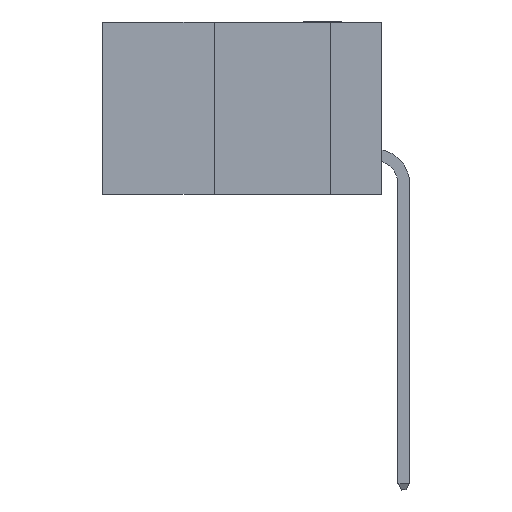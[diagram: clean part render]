
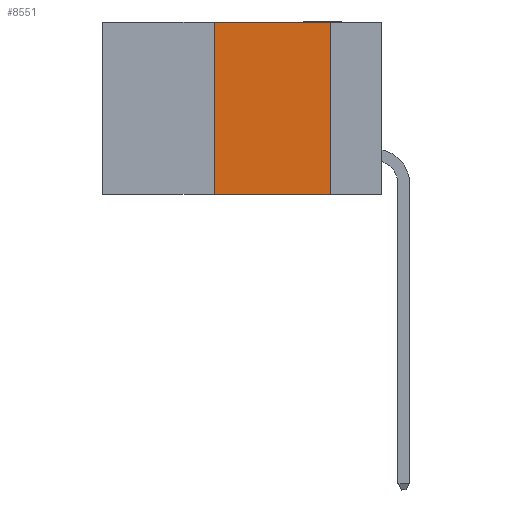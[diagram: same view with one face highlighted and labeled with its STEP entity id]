
A CAD part, left-side view. The second image highlights one B-rep face of the part: STEP entity #8551.
In plain terms, the highlighted planar face has unit normal (-1, 0, 0).
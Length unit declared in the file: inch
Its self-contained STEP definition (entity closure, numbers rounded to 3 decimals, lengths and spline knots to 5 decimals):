
#49 = VECTOR ( 'NONE', #8994, 39.37008 ) ;
#125 = ORIENTED_EDGE ( 'NONE', *, *, #8470, .F. ) ;
#717 = DIRECTION ( 'NONE',  ( 0., 0., 1. ) ) ;
#779 = LINE ( 'NONE', #12101, #2679 ) ;
#1007 = EDGE_LOOP ( 'NONE', ( #125, #6631, #2902, #10800 ) ) ;
#1038 = FACE_OUTER_BOUND ( 'NONE', #1007, .T. ) ;
#1127 = LINE ( 'NONE', #4675, #7834 ) ;
#1640 = DIRECTION ( 'NONE',  ( 0., -1., 0. ) ) ;
#1758 = CARTESIAN_POINT ( 'NONE',  ( 0., 0.6, -0.37 ) ) ;
#1955 = VECTOR ( 'NONE', #12818, 39.37008 ) ;
#2222 = VERTEX_POINT ( 'NONE', #10790 ) ;
#2679 = VECTOR ( 'NONE', #717, 39.37008 ) ;
#2902 = ORIENTED_EDGE ( 'NONE', *, *, #9656, .F. ) ;
#3078 = LINE ( 'NONE', #1758, #49 ) ;
#3686 = CARTESIAN_POINT ( 'NONE',  ( 0., 0.11, 0. ) ) ;
#3715 = LINE ( 'NONE', #3686, #1955 ) ;
#4675 = CARTESIAN_POINT ( 'NONE',  ( 0., 0.6, 0. ) ) ;
#5022 = EDGE_CURVE ( 'NONE', #2222, #8642, #1127, .T. ) ;
#5127 = DIRECTION ( 'NONE',  ( 0., 0., -1. ) ) ;
#6254 = CARTESIAN_POINT ( 'NONE',  ( 0., 0.11, 0. ) ) ;
#6631 = ORIENTED_EDGE ( 'NONE', *, *, #5022, .F. ) ;
#7381 = VERTEX_POINT ( 'NONE', #9465 ) ;
#7790 = CARTESIAN_POINT ( 'NONE',  ( 0., 0.11, -0.37 ) ) ;
#7834 = VECTOR ( 'NONE', #1640, 39.37008 ) ;
#8470 = EDGE_CURVE ( 'NONE', #8642, #12181, #3715, .T. ) ;
#8551 = ADVANCED_FACE ( 'NONE', ( #1038 ), #11294, .F. ) ;
#8642 = VERTEX_POINT ( 'NONE', #6254 ) ;
#8994 = DIRECTION ( 'NONE',  ( 0., -1., 0. ) ) ;
#9150 = CARTESIAN_POINT ( 'NONE',  ( 0., 0.6, 0. ) ) ;
#9465 = CARTESIAN_POINT ( 'NONE',  ( 0., 0.36, -0.37 ) ) ;
#9656 = EDGE_CURVE ( 'NONE', #7381, #2222, #779, .T. ) ;
#10790 = CARTESIAN_POINT ( 'NONE',  ( 0., 0.36, 0. ) ) ;
#10800 = ORIENTED_EDGE ( 'NONE', *, *, #12924, .T. ) ;
#11294 = PLANE ( 'NONE',  #12787 ) ;
#11329 = DIRECTION ( 'NONE',  ( 1., 0., 0. ) ) ;
#12101 = CARTESIAN_POINT ( 'NONE',  ( 0., 0.36, 0. ) ) ;
#12181 = VERTEX_POINT ( 'NONE', #7790 ) ;
#12787 = AXIS2_PLACEMENT_3D ( 'NONE', #9150, #11329, #5127 ) ;
#12818 = DIRECTION ( 'NONE',  ( 0., 0., -1. ) ) ;
#12924 = EDGE_CURVE ( 'NONE', #7381, #12181, #3078, .T. ) ;
